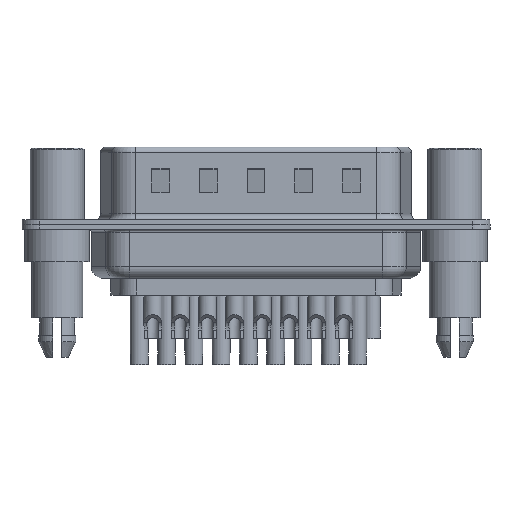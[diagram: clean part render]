
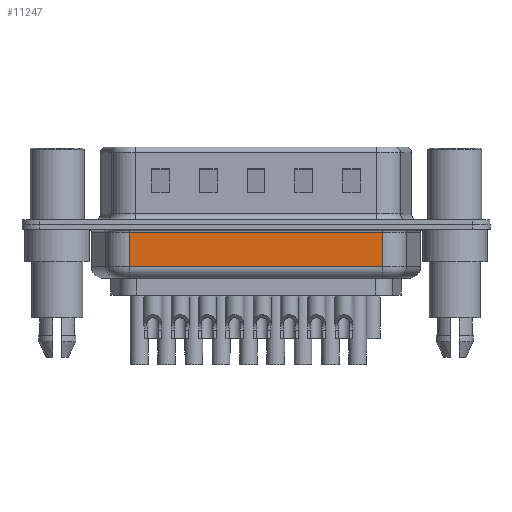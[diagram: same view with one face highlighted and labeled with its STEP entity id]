
A CAD part, front view. The second image highlights one B-rep face of the part: STEP entity #11247.
In plain terms, the highlighted planar face has unit normal (0, -1, 0).
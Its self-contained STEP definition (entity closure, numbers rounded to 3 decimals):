
#14 = DIRECTION ( 'NONE',  ( -1., 0., 0. ) ) ;
#46 = VERTEX_POINT ( 'NONE', #21334 ) ;
#891 = VECTOR ( 'NONE', #19010, 1000. ) ;
#2509 = VECTOR ( 'NONE', #13690, 1000. ) ;
#2857 = AXIS2_PLACEMENT_3D ( 'NONE', #20133, #10125, #14 ) ;
#3597 = VECTOR ( 'NONE', #20314, 1000. ) ;
#3735 = LINE ( 'NONE', #6862, #7672 ) ;
#3970 = CARTESIAN_POINT ( 'NONE',  ( 6.031, -5.35, -3.5 ) ) ;
#4130 = LINE ( 'NONE', #12001, #3597 ) ;
#4854 = EDGE_CURVE ( 'NONE', #15692, #7888, #20279, .T. ) ;
#5157 = DIRECTION ( 'NONE',  ( 0., 0., 1. ) ) ;
#5764 = ORIENTED_EDGE ( 'NONE', *, *, #21114, .T. ) ;
#6862 = CARTESIAN_POINT ( 'NONE',  ( 27.269, -5.35, -4.5 ) ) ;
#7672 = VECTOR ( 'NONE', #5157, 1000. ) ;
#7888 = VERTEX_POINT ( 'NONE', #10107 ) ;
#8526 = EDGE_CURVE ( 'NONE', #19936, #7888, #4130, .T. ) ;
#9340 = CARTESIAN_POINT ( 'NONE',  ( 6.031, -5.35, -3.5 ) ) ;
#9534 = CARTESIAN_POINT ( 'NONE',  ( 6.031, -5.35, -4.5 ) ) ;
#10107 = CARTESIAN_POINT ( 'NONE',  ( 6.031, -5.35, -0.65 ) ) ;
#10125 = DIRECTION ( 'NONE',  ( 0., 1., 0. ) ) ;
#11247 = ADVANCED_FACE ( 'NONE', ( #12724 ), #16717, .F. ) ;
#12001 = CARTESIAN_POINT ( 'NONE',  ( 6.031, -5.35, -0.65 ) ) ;
#12293 = ORIENTED_EDGE ( 'NONE', *, *, #4854, .F. ) ;
#12724 = FACE_OUTER_BOUND ( 'NONE', #18838, .T. ) ;
#13690 = DIRECTION ( 'NONE',  ( 0., 0., 1. ) ) ;
#14397 = ORIENTED_EDGE ( 'NONE', *, *, #18021, .T. ) ;
#15692 = VERTEX_POINT ( 'NONE', #9340 ) ;
#16717 = PLANE ( 'NONE',  #2857 ) ;
#18021 = EDGE_CURVE ( 'NONE', #15692, #46, #18711, .T. ) ;
#18672 = CARTESIAN_POINT ( 'NONE',  ( 27.269, -5.35, -0.65 ) ) ;
#18711 = LINE ( 'NONE', #3970, #891 ) ;
#18838 = EDGE_LOOP ( 'NONE', ( #12293, #14397, #5764, #19044 ) ) ;
#19010 = DIRECTION ( 'NONE',  ( 1., 0., 0. ) ) ;
#19044 = ORIENTED_EDGE ( 'NONE', *, *, #8526, .T. ) ;
#19936 = VERTEX_POINT ( 'NONE', #18672 ) ;
#20133 = CARTESIAN_POINT ( 'NONE',  ( 6.031, -5.35, -4.5 ) ) ;
#20279 = LINE ( 'NONE', #9534, #2509 ) ;
#20314 = DIRECTION ( 'NONE',  ( -1., 0., 0. ) ) ;
#21114 = EDGE_CURVE ( 'NONE', #46, #19936, #3735, .T. ) ;
#21334 = CARTESIAN_POINT ( 'NONE',  ( 27.269, -5.35, -3.5 ) ) ;
